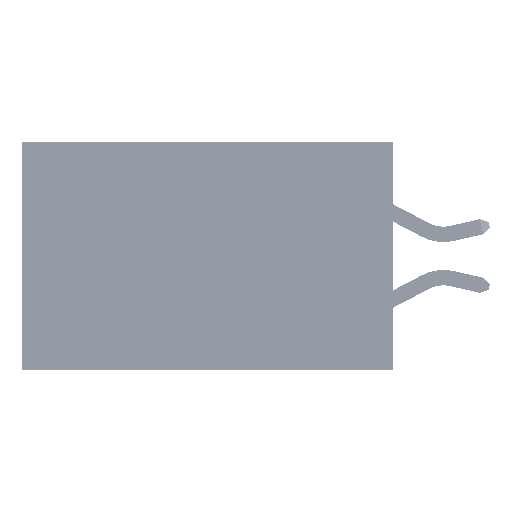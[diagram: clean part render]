
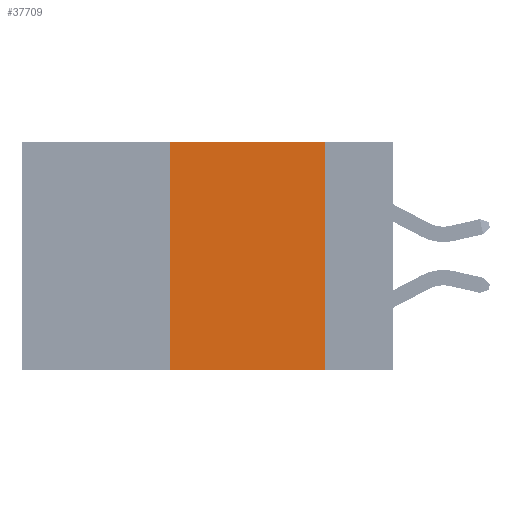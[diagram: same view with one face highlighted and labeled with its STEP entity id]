
A CAD part, left-side view. The second image highlights one B-rep face of the part: STEP entity #37709.
In plain terms, the highlighted planar face has unit normal (-1, 0, 0).
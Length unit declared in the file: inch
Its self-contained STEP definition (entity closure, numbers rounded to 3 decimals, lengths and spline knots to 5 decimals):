
#1800 = FACE_OUTER_BOUND ( 'NONE', #35133, .T. ) ;
#2896 = VERTEX_POINT ( 'NONE', #20991 ) ;
#5208 = EDGE_CURVE ( 'NONE', #13047, #16189, #46941, .T. ) ;
#5784 = ORIENTED_EDGE ( 'NONE', *, *, #44238, .T. ) ;
#6720 = ORIENTED_EDGE ( 'NONE', *, *, #28838, .F. ) ;
#6733 = EDGE_CURVE ( 'NONE', #16189, #45781, #41943, .T. ) ;
#7840 = CARTESIAN_POINT ( 'NONE',  ( 0., 0.36, 0. ) ) ;
#8268 = CARTESIAN_POINT ( 'NONE',  ( 0., 0.11, 0. ) ) ;
#9384 = LINE ( 'NONE', #26114, #14236 ) ;
#10664 = DIRECTION ( 'NONE',  ( 0., -1., 0. ) ) ;
#13047 = VERTEX_POINT ( 'NONE', #46465 ) ;
#13178 = AXIS2_PLACEMENT_3D ( 'NONE', #14017, #41138, #29825 ) ;
#14017 = CARTESIAN_POINT ( 'NONE',  ( 0., 0.6, 0. ) ) ;
#14236 = VECTOR ( 'NONE', #10664, 39.37008 ) ;
#15296 = VECTOR ( 'NONE', #23512, 39.37008 ) ;
#16189 = VERTEX_POINT ( 'NONE', #7840 ) ;
#16303 = DIRECTION ( 'NONE',  ( 0., 0., 1. ) ) ;
#20991 = CARTESIAN_POINT ( 'NONE',  ( 0., 0.11, -0.37 ) ) ;
#21005 = VECTOR ( 'NONE', #35905, 39.37008 ) ;
#22722 = VECTOR ( 'NONE', #16303, 39.37008 ) ;
#23329 = CARTESIAN_POINT ( 'NONE',  ( 0., 0.6, 0. ) ) ;
#23512 = DIRECTION ( 'NONE',  ( 0., -1., 0. ) ) ;
#26114 = CARTESIAN_POINT ( 'NONE',  ( 0., 0.6, -0.37 ) ) ;
#28838 = EDGE_CURVE ( 'NONE', #45781, #2896, #45223, .T. ) ;
#29825 = DIRECTION ( 'NONE',  ( 0., 0., -1. ) ) ;
#33536 = ORIENTED_EDGE ( 'NONE', *, *, #5208, .F. ) ;
#35133 = EDGE_LOOP ( 'NONE', ( #6720, #48150, #33536, #5784 ) ) ;
#35905 = DIRECTION ( 'NONE',  ( 0., 0., -1. ) ) ;
#37261 = PLANE ( 'NONE',  #13178 ) ;
#37709 = ADVANCED_FACE ( 'NONE', ( #1800 ), #37261, .F. ) ;
#39144 = CARTESIAN_POINT ( 'NONE',  ( 0., 0.11, 0. ) ) ;
#41138 = DIRECTION ( 'NONE',  ( 1., 0., 0. ) ) ;
#41943 = LINE ( 'NONE', #23329, #15296 ) ;
#44238 = EDGE_CURVE ( 'NONE', #13047, #2896, #9384, .T. ) ;
#45223 = LINE ( 'NONE', #8268, #21005 ) ;
#45781 = VERTEX_POINT ( 'NONE', #39144 ) ;
#46465 = CARTESIAN_POINT ( 'NONE',  ( 0., 0.36, -0.37 ) ) ;
#46799 = CARTESIAN_POINT ( 'NONE',  ( 0., 0.36, 0. ) ) ;
#46941 = LINE ( 'NONE', #46799, #22722 ) ;
#48150 = ORIENTED_EDGE ( 'NONE', *, *, #6733, .F. ) ;
